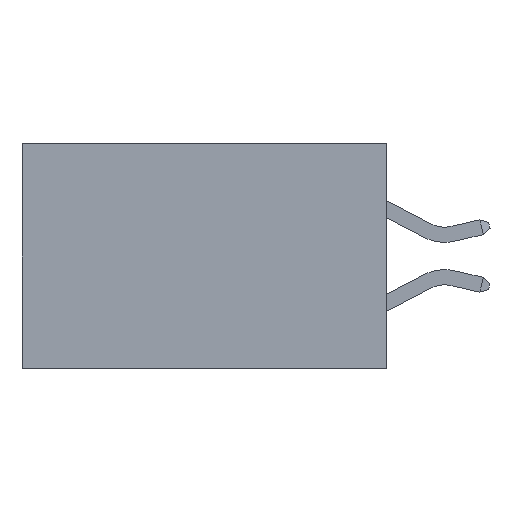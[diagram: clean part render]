
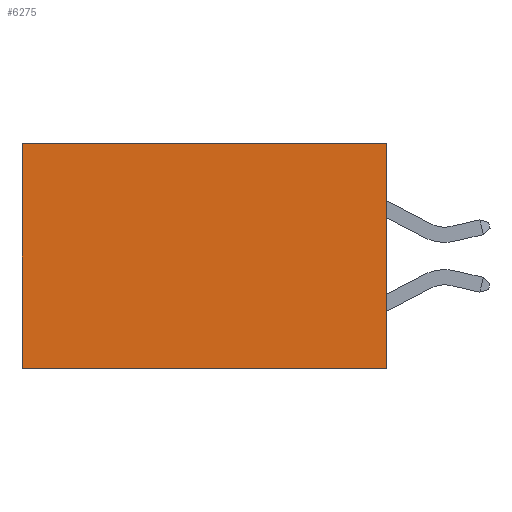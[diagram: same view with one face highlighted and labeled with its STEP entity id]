
A CAD part, left-side view. The second image highlights one B-rep face of the part: STEP entity #6275.
In plain terms, the highlighted planar face has unit normal (-1, 0, 0).
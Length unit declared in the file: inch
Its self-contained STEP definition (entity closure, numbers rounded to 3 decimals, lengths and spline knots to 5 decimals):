
#337 = EDGE_CURVE ( 'NONE', #5368, #1198, #7116, .T. ) ;
#366 = LINE ( 'NONE', #10843, #7218 ) ;
#483 = CARTESIAN_POINT ( 'NONE',  ( 0.2615, 0., -0.37 ) ) ;
#659 = DIRECTION ( 'NONE',  ( 0., 0., -1. ) ) ;
#855 = VECTOR ( 'NONE', #9791, 39.37008 ) ;
#1053 = ORIENTED_EDGE ( 'NONE', *, *, #9375, .T. ) ;
#1198 = VERTEX_POINT ( 'NONE', #7091 ) ;
#1765 = CARTESIAN_POINT ( 'NONE',  ( 0.2615, 0., -0.37 ) ) ;
#1785 = DIRECTION ( 'NONE',  ( 0., 0., -1. ) ) ;
#2174 = DIRECTION ( 'NONE',  ( 0., 1., 0. ) ) ;
#2546 = PLANE ( 'NONE',  #4001 ) ;
#2602 = CARTESIAN_POINT ( 'NONE',  ( 0.2615, 0., -0.37 ) ) ;
#4001 = AXIS2_PLACEMENT_3D ( 'NONE', #2602, #9798, #7176 ) ;
#5074 = ORIENTED_EDGE ( 'NONE', *, *, #337, .T. ) ;
#5368 = VERTEX_POINT ( 'NONE', #8166 ) ;
#5536 = CARTESIAN_POINT ( 'NONE',  ( 0.2615, 0., 0. ) ) ;
#6060 = VECTOR ( 'NONE', #1785, 39.37008 ) ;
#6238 = LINE ( 'NONE', #5536, #855 ) ;
#6275 = ADVANCED_FACE ( 'NONE', ( #10634 ), #2546, .F. ) ;
#6752 = LINE ( 'NONE', #483, #6881 ) ;
#6762 = VERTEX_POINT ( 'NONE', #1765 ) ;
#6881 = VECTOR ( 'NONE', #659, 39.37008 ) ;
#7091 = CARTESIAN_POINT ( 'NONE',  ( 0.2615, 0.6, -0.37 ) ) ;
#7116 = LINE ( 'NONE', #9026, #6060 ) ;
#7169 = CARTESIAN_POINT ( 'NONE',  ( 0.2615, 0., 0. ) ) ;
#7176 = DIRECTION ( 'NONE',  ( 0., 0., -1. ) ) ;
#7218 = VECTOR ( 'NONE', #2174, 39.37008 ) ;
#8166 = CARTESIAN_POINT ( 'NONE',  ( 0.2615, 0.6, 0. ) ) ;
#8622 = ORIENTED_EDGE ( 'NONE', *, *, #10051, .F. ) ;
#9026 = CARTESIAN_POINT ( 'NONE',  ( 0.2615, 0.6, -0.37 ) ) ;
#9269 = VERTEX_POINT ( 'NONE', #7169 ) ;
#9375 = EDGE_CURVE ( 'NONE', #9269, #5368, #6238, .T. ) ;
#9782 = EDGE_LOOP ( 'NONE', ( #5074, #8622, #10447, #1053 ) ) ;
#9791 = DIRECTION ( 'NONE',  ( 0., 1., 0. ) ) ;
#9798 = DIRECTION ( 'NONE',  ( 1., 0., 0. ) ) ;
#10051 = EDGE_CURVE ( 'NONE', #6762, #1198, #366, .T. ) ;
#10447 = ORIENTED_EDGE ( 'NONE', *, *, #11535, .F. ) ;
#10634 = FACE_OUTER_BOUND ( 'NONE', #9782, .T. ) ;
#10843 = CARTESIAN_POINT ( 'NONE',  ( 0.2615, 0., -0.37 ) ) ;
#11535 = EDGE_CURVE ( 'NONE', #9269, #6762, #6752, .T. ) ;
